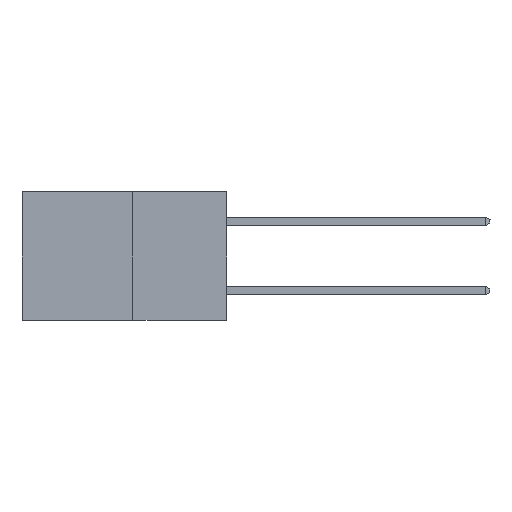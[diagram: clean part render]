
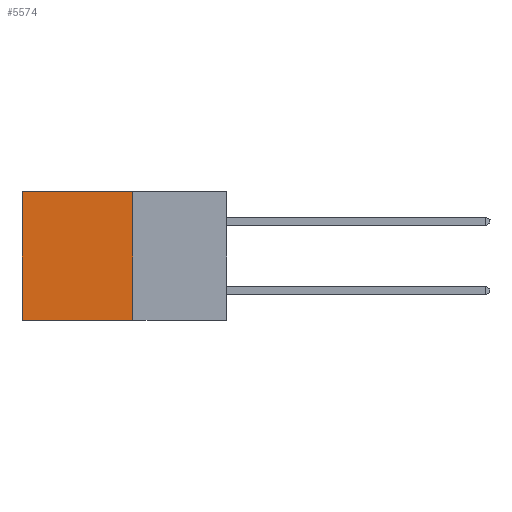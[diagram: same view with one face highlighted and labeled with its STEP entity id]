
A CAD part, left-side view. The second image highlights one B-rep face of the part: STEP entity #5574.
In plain terms, the highlighted planar face has unit normal (-1, 0, 0).
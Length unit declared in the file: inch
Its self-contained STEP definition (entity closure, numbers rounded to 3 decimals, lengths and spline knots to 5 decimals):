
#579 = DIRECTION ( 'NONE',  ( 0., 1., 0. ) ) ;
#939 = AXIS2_PLACEMENT_3D ( 'NONE', #23368, #2464, #2046 ) ;
#1811 = EDGE_CURVE ( 'NONE', #4842, #9477, #23759, .T. ) ;
#1956 = CARTESIAN_POINT ( 'NONE',  ( 0.277, 0.59, 0. ) ) ;
#2046 = DIRECTION ( 'NONE',  ( 0., 0., -1. ) ) ;
#2464 = DIRECTION ( 'NONE',  ( 1., 0., 0. ) ) ;
#4842 = VERTEX_POINT ( 'NONE', #4874 ) ;
#4844 = EDGE_CURVE ( 'NONE', #9477, #28122, #14662, .T. ) ;
#4874 = CARTESIAN_POINT ( 'NONE',  ( 0.277, 0.27, 0. ) ) ;
#5328 = CARTESIAN_POINT ( 'NONE',  ( 0.277, 0.59, -0.37 ) ) ;
#5574 = ADVANCED_FACE ( 'NONE', ( #33208 ), #23806, .F. ) ;
#7035 = ORIENTED_EDGE ( 'NONE', *, *, #30950, .F. ) ;
#7723 = VECTOR ( 'NONE', #15846, 39.37008 ) ;
#9477 = VERTEX_POINT ( 'NONE', #1956 ) ;
#12417 = CARTESIAN_POINT ( 'NONE',  ( 0.277, 0.27, -0.37 ) ) ;
#13359 = ORIENTED_EDGE ( 'NONE', *, *, #4844, .T. ) ;
#14662 = LINE ( 'NONE', #5328, #7723 ) ;
#15846 = DIRECTION ( 'NONE',  ( 0., 0., -1. ) ) ;
#15980 = ORIENTED_EDGE ( 'NONE', *, *, #1811, .T. ) ;
#16757 = VECTOR ( 'NONE', #25327, 39.37008 ) ;
#16838 = CARTESIAN_POINT ( 'NONE',  ( 0.277, 0.27, 0. ) ) ;
#17690 = EDGE_CURVE ( 'NONE', #26863, #28122, #32046, .T. ) ;
#18266 = VECTOR ( 'NONE', #579, 39.37008 ) ;
#20724 = CARTESIAN_POINT ( 'NONE',  ( 0.277, 0.59, -0.37 ) ) ;
#23065 = CARTESIAN_POINT ( 'NONE',  ( 0.277, 0.27, -0.37 ) ) ;
#23368 = CARTESIAN_POINT ( 'NONE',  ( 0.277, 0.27, -0.37 ) ) ;
#23618 = LINE ( 'NONE', #12417, #16757 ) ;
#23759 = LINE ( 'NONE', #16838, #24589 ) ;
#23802 = DIRECTION ( 'NONE',  ( 0., 1., 0. ) ) ;
#23806 = PLANE ( 'NONE',  #939 ) ;
#24589 = VECTOR ( 'NONE', #23802, 39.37008 ) ;
#25327 = DIRECTION ( 'NONE',  ( 0., 0., -1. ) ) ;
#25773 = EDGE_LOOP ( 'NONE', ( #13359, #32284, #7035, #15980 ) ) ;
#26863 = VERTEX_POINT ( 'NONE', #23065 ) ;
#28122 = VERTEX_POINT ( 'NONE', #20724 ) ;
#30950 = EDGE_CURVE ( 'NONE', #4842, #26863, #23618, .T. ) ;
#31767 = CARTESIAN_POINT ( 'NONE',  ( 0.277, 0.27, -0.37 ) ) ;
#32046 = LINE ( 'NONE', #31767, #18266 ) ;
#32284 = ORIENTED_EDGE ( 'NONE', *, *, #17690, .F. ) ;
#33208 = FACE_OUTER_BOUND ( 'NONE', #25773, .T. ) ;
